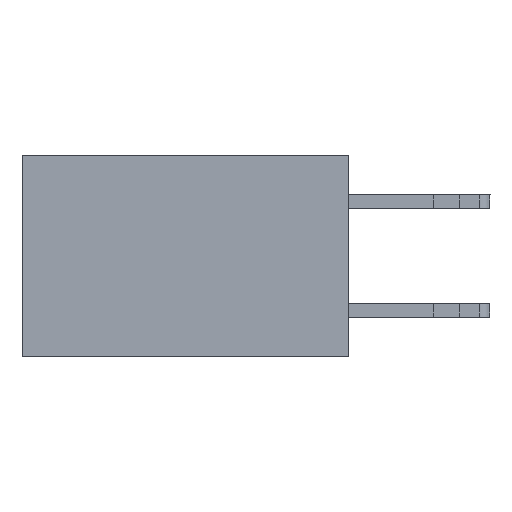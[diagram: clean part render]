
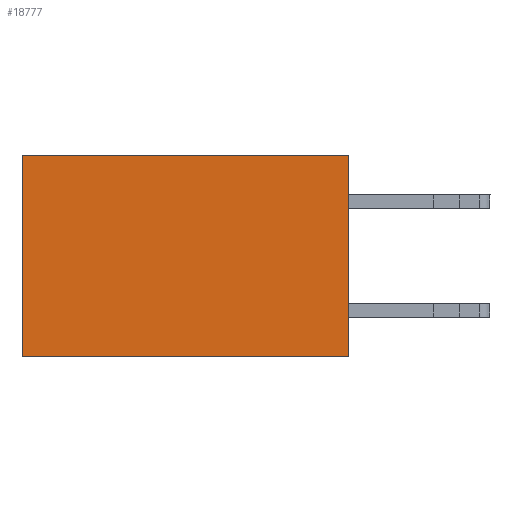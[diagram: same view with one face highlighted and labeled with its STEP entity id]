
A CAD part, left-side view. The second image highlights one B-rep face of the part: STEP entity #18777.
In plain terms, the highlighted planar face has unit normal (-1, 0, 0).
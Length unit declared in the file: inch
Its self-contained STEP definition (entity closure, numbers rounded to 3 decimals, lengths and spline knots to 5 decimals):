
#218 = FACE_OUTER_BOUND ( 'NONE', #3281, .T. ) ;
#902 = ORIENTED_EDGE ( 'NONE', *, *, #1508, .F. ) ;
#1170 = ORIENTED_EDGE ( 'NONE', *, *, #23079, .T. ) ;
#1508 = EDGE_CURVE ( 'NONE', #27584, #12768, #18930, .T. ) ;
#1678 = CARTESIAN_POINT ( 'NONE',  ( 0.298, 0., -0.37 ) ) ;
#3281 = EDGE_LOOP ( 'NONE', ( #24641, #902, #12504, #1170 ) ) ;
#3390 = DIRECTION ( 'NONE',  ( 0., 0., -1. ) ) ;
#4091 = VECTOR ( 'NONE', #16820, 39.37008 ) ;
#5170 = LINE ( 'NONE', #7386, #13557 ) ;
#6638 = DIRECTION ( 'NONE',  ( 1., 0., 0. ) ) ;
#6925 = CARTESIAN_POINT ( 'NONE',  ( 0.298, 0., 0. ) ) ;
#6982 = CARTESIAN_POINT ( 'NONE',  ( 0.298, 0.6, 0. ) ) ;
#7386 = CARTESIAN_POINT ( 'NONE',  ( 0.298, 0.6, 0. ) ) ;
#12366 = CARTESIAN_POINT ( 'NONE',  ( 0.298, 0.6, -0.37 ) ) ;
#12504 = ORIENTED_EDGE ( 'NONE', *, *, #13647, .F. ) ;
#12697 = VECTOR ( 'NONE', #13561, 39.37008 ) ;
#12768 = VERTEX_POINT ( 'NONE', #12366 ) ;
#12972 = EDGE_CURVE ( 'NONE', #23218, #12768, #5170, .T. ) ;
#13465 = CARTESIAN_POINT ( 'NONE',  ( 0.298, 0., -0.37 ) ) ;
#13557 = VECTOR ( 'NONE', #3390, 39.37008 ) ;
#13561 = DIRECTION ( 'NONE',  ( 0., 0., -1. ) ) ;
#13647 = EDGE_CURVE ( 'NONE', #17069, #27584, #17332, .T. ) ;
#14491 = CARTESIAN_POINT ( 'NONE',  ( 0.298, 0., 0. ) ) ;
#15277 = DIRECTION ( 'NONE',  ( 0., 0., -1. ) ) ;
#16820 = DIRECTION ( 'NONE',  ( 0., 1., 0. ) ) ;
#17069 = VERTEX_POINT ( 'NONE', #14491 ) ;
#17332 = LINE ( 'NONE', #6925, #12697 ) ;
#17334 = PLANE ( 'NONE',  #18527 ) ;
#18527 = AXIS2_PLACEMENT_3D ( 'NONE', #25922, #6638, #15277 ) ;
#18777 = ADVANCED_FACE ( 'NONE', ( #218 ), #17334, .F. ) ;
#18930 = LINE ( 'NONE', #1678, #4091 ) ;
#23079 = EDGE_CURVE ( 'NONE', #17069, #23218, #26027, .T. ) ;
#23218 = VERTEX_POINT ( 'NONE', #6982 ) ;
#24330 = CARTESIAN_POINT ( 'NONE',  ( 0.298, 0., 0. ) ) ;
#24641 = ORIENTED_EDGE ( 'NONE', *, *, #12972, .T. ) ;
#25922 = CARTESIAN_POINT ( 'NONE',  ( 0.298, 0., 0. ) ) ;
#26018 = VECTOR ( 'NONE', #26175, 39.37008 ) ;
#26027 = LINE ( 'NONE', #24330, #26018 ) ;
#26175 = DIRECTION ( 'NONE',  ( 0., 1., 0. ) ) ;
#27584 = VERTEX_POINT ( 'NONE', #13465 ) ;
